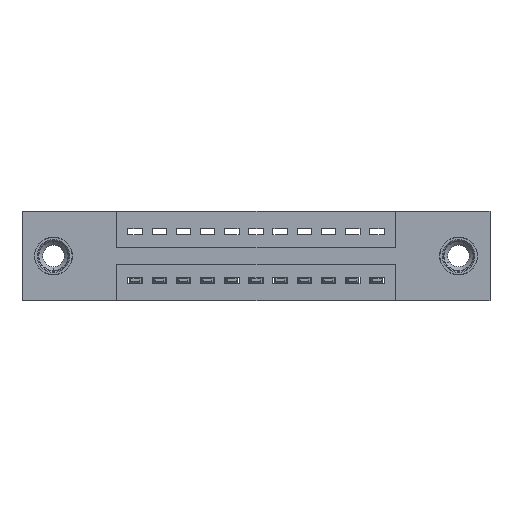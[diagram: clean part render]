
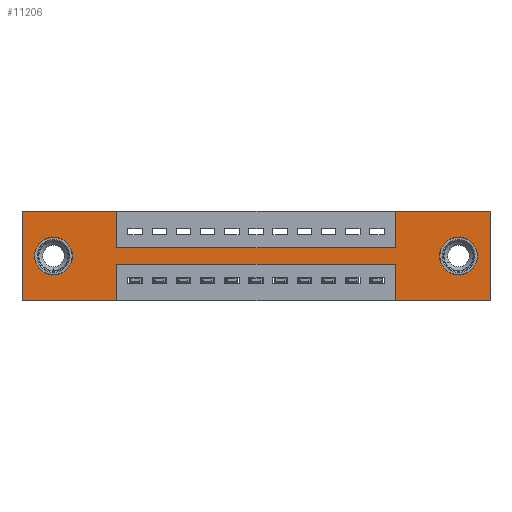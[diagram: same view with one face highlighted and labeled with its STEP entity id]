
A CAD part, front view. The second image highlights one B-rep face of the part: STEP entity #11206.
In plain terms, the highlighted planar face has unit normal (0, -1, 0).
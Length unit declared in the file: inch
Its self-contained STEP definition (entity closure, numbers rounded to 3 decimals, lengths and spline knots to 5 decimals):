
#356 = DIRECTION ( 'NONE',  ( -1., 0., 0. ) ) ;
#360 = ORIENTED_EDGE ( 'NONE', *, *, #8458, .F. ) ;
#380 = LINE ( 'NONE', #4766, #1817 ) ;
#430 = DIRECTION ( 'NONE',  ( 0., 1., 0. ) ) ;
#636 = ORIENTED_EDGE ( 'NONE', *, *, #5639, .F. ) ;
#683 = DIRECTION ( 'NONE',  ( 0., 0., -1. ) ) ;
#984 = CARTESIAN_POINT ( 'NONE',  ( 0.13, 0., -0.263 ) ) ;
#1240 = VERTEX_POINT ( 'NONE', #5807 ) ;
#1461 = VERTEX_POINT ( 'NONE', #5908 ) ;
#1475 = ORIENTED_EDGE ( 'NONE', *, *, #4261, .F. ) ;
#1483 = LINE ( 'NONE', #5819, #6664 ) ;
#1589 = EDGE_CURVE ( 'NONE', #9004, #10966, #3359, .T. ) ;
#1738 = VECTOR ( 'NONE', #13070, 39.37008 ) ;
#1817 = VECTOR ( 'NONE', #9837, 39.37008 ) ;
#1819 = EDGE_CURVE ( 'NONE', #8498, #11191, #4679, .T. ) ;
#1848 = FACE_BOUND ( 'NONE', #7551, .T. ) ;
#1968 = LINE ( 'NONE', #8083, #6820 ) ;
#1998 = ORIENTED_EDGE ( 'NONE', *, *, #6549, .F. ) ;
#2251 = VERTEX_POINT ( 'NONE', #9491 ) ;
#2304 = CARTESIAN_POINT ( 'NONE',  ( 0.3925, 0., -0.22 ) ) ;
#2522 = FACE_BOUND ( 'NONE', #7835, .T. ) ;
#2549 = VERTEX_POINT ( 'NONE', #10984 ) ;
#2738 = CARTESIAN_POINT ( 'NONE',  ( 1.935, 0., 0. ) ) ;
#3197 = PLANE ( 'NONE',  #4906 ) ;
#3282 = DIRECTION ( 'NONE',  ( -1., 0., 0. ) ) ;
#3312 = LINE ( 'NONE', #2304, #10624 ) ;
#3359 = LINE ( 'NONE', #5860, #1738 ) ;
#3496 = CARTESIAN_POINT ( 'NONE',  ( 1.805, 0., -0.107 ) ) ;
#3548 = DIRECTION ( 'NONE',  ( 0., 0., 1. ) ) ;
#3571 = ORIENTED_EDGE ( 'NONE', *, *, #1589, .F. ) ;
#4129 = CIRCLE ( 'NONE', #7503, 0.078 ) ;
#4219 = CARTESIAN_POINT ( 'NONE',  ( 0., 0., -0.37 ) ) ;
#4261 = EDGE_CURVE ( 'NONE', #1461, #6462, #380, .T. ) ;
#4270 = DIRECTION ( 'NONE',  ( 0., -1., 0. ) ) ;
#4402 = CARTESIAN_POINT ( 'NONE',  ( 0.3925, 0., 0. ) ) ;
#4442 = VECTOR ( 'NONE', #5449, 39.37008 ) ;
#4548 = DIRECTION ( 'NONE',  ( 0., 0., -1. ) ) ;
#4679 = CIRCLE ( 'NONE', #10626, 0.078 ) ;
#4725 = VECTOR ( 'NONE', #4548, 39.37008 ) ;
#4766 = CARTESIAN_POINT ( 'NONE',  ( 0., 0., 0. ) ) ;
#4904 = ORIENTED_EDGE ( 'NONE', *, *, #4978, .T. ) ;
#4906 = AXIS2_PLACEMENT_3D ( 'NONE', #10475, #4270, #11532 ) ;
#4953 = VECTOR ( 'NONE', #356, 39.37008 ) ;
#4954 = VECTOR ( 'NONE', #12612, 39.37008 ) ;
#4967 = CIRCLE ( 'NONE', #12934, 0.078 ) ;
#4978 = EDGE_CURVE ( 'NONE', #10634, #2251, #4129, .T. ) ;
#5097 = VERTEX_POINT ( 'NONE', #6298 ) ;
#5151 = CARTESIAN_POINT ( 'NONE',  ( 1.805, 0., -0.263 ) ) ;
#5184 = VERTEX_POINT ( 'NONE', #11077 ) ;
#5257 = DIRECTION ( 'NONE',  ( 0., 0., 1. ) ) ;
#5449 = DIRECTION ( 'NONE',  ( 0., 0., -1. ) ) ;
#5511 = ORIENTED_EDGE ( 'NONE', *, *, #7970, .F. ) ;
#5639 = EDGE_CURVE ( 'NONE', #10966, #6161, #13243, .T. ) ;
#5807 = CARTESIAN_POINT ( 'NONE',  ( 1.5425, 0., -0.37 ) ) ;
#5819 = CARTESIAN_POINT ( 'NONE',  ( 0., 0., 0. ) ) ;
#5829 = ORIENTED_EDGE ( 'NONE', *, *, #12043, .T. ) ;
#5836 = LINE ( 'NONE', #10740, #4725 ) ;
#5860 = CARTESIAN_POINT ( 'NONE',  ( 0.3925, 0., -0.37 ) ) ;
#5908 = CARTESIAN_POINT ( 'NONE',  ( 0., 0., 0. ) ) ;
#6161 = VERTEX_POINT ( 'NONE', #8451 ) ;
#6214 = LINE ( 'NONE', #4219, #4954 ) ;
#6296 = VERTEX_POINT ( 'NONE', #7533 ) ;
#6298 = CARTESIAN_POINT ( 'NONE',  ( 1.935, 0., -0.37 ) ) ;
#6394 = ORIENTED_EDGE ( 'NONE', *, *, #7751, .F. ) ;
#6450 = LINE ( 'NONE', #9413, #8413 ) ;
#6462 = VERTEX_POINT ( 'NONE', #11830 ) ;
#6549 = EDGE_CURVE ( 'NONE', #6161, #1461, #1968, .T. ) ;
#6664 = VECTOR ( 'NONE', #13110, 39.37008 ) ;
#6765 = VECTOR ( 'NONE', #5257, 39.37008 ) ;
#6820 = VECTOR ( 'NONE', #9135, 39.37008 ) ;
#6829 = ORIENTED_EDGE ( 'NONE', *, *, #9706, .F. ) ;
#7006 = EDGE_CURVE ( 'NONE', #2251, #10634, #13032, .T. ) ;
#7265 = CARTESIAN_POINT ( 'NONE',  ( 1.5425, 0., 0. ) ) ;
#7373 = ORIENTED_EDGE ( 'NONE', *, *, #13095, .F. ) ;
#7503 = AXIS2_PLACEMENT_3D ( 'NONE', #12890, #430, #3548 ) ;
#7533 = CARTESIAN_POINT ( 'NONE',  ( 1.5425, 0., 0. ) ) ;
#7551 = EDGE_LOOP ( 'NONE', ( #10809, #4904 ) ) ;
#7616 = DIRECTION ( 'NONE',  ( 0., 1., 0. ) ) ;
#7644 = EDGE_LOOP ( 'NONE', ( #3571, #11677, #6829, #8722, #6394, #7373, #360, #5511, #10384, #1475, #1998, #636 ) ) ;
#7751 = EDGE_CURVE ( 'NONE', #11159, #5097, #5836, .T. ) ;
#7835 = EDGE_LOOP ( 'NONE', ( #13031, #5829 ) ) ;
#7970 = EDGE_CURVE ( 'NONE', #5184, #12157, #6450, .T. ) ;
#8083 = CARTESIAN_POINT ( 'NONE',  ( 0., 0., 0. ) ) ;
#8365 = VECTOR ( 'NONE', #11875, 39.37008 ) ;
#8413 = VECTOR ( 'NONE', #10231, 39.37008 ) ;
#8451 = CARTESIAN_POINT ( 'NONE',  ( 0., 0., -0.37 ) ) ;
#8458 = EDGE_CURVE ( 'NONE', #12157, #6296, #11837, .T. ) ;
#8498 = VERTEX_POINT ( 'NONE', #3496 ) ;
#8528 = DIRECTION ( 'NONE',  ( 0., 0., -1. ) ) ;
#8722 = ORIENTED_EDGE ( 'NONE', *, *, #12394, .F. ) ;
#8934 = CARTESIAN_POINT ( 'NONE',  ( 1.5425, 0., -0.15 ) ) ;
#9004 = VERTEX_POINT ( 'NONE', #13440 ) ;
#9135 = DIRECTION ( 'NONE',  ( 0., 0., 1. ) ) ;
#9413 = CARTESIAN_POINT ( 'NONE',  ( 0.3925, 0., -0.15 ) ) ;
#9451 = CARTESIAN_POINT ( 'NONE',  ( 0.13, 0., -0.185 ) ) ;
#9491 = CARTESIAN_POINT ( 'NONE',  ( 0.13, 0., -0.107 ) ) ;
#9600 = CARTESIAN_POINT ( 'NONE',  ( 0.3925, 0., -0.37 ) ) ;
#9706 = EDGE_CURVE ( 'NONE', #1240, #2549, #12804, .T. ) ;
#9837 = DIRECTION ( 'NONE',  ( 1., 0., 0. ) ) ;
#9955 = CARTESIAN_POINT ( 'NONE',  ( 1.5425, 0., -0.37 ) ) ;
#10231 = DIRECTION ( 'NONE',  ( 1., 0., 0. ) ) ;
#10384 = ORIENTED_EDGE ( 'NONE', *, *, #12598, .F. ) ;
#10475 = CARTESIAN_POINT ( 'NONE',  ( 0., 0., -0.37 ) ) ;
#10624 = VECTOR ( 'NONE', #3282, 39.37008 ) ;
#10626 = AXIS2_PLACEMENT_3D ( 'NONE', #11067, #10929, #683 ) ;
#10634 = VERTEX_POINT ( 'NONE', #984 ) ;
#10740 = CARTESIAN_POINT ( 'NONE',  ( 1.935, 0., 0. ) ) ;
#10809 = ORIENTED_EDGE ( 'NONE', *, *, #7006, .T. ) ;
#10870 = EDGE_CURVE ( 'NONE', #2549, #9004, #3312, .T. ) ;
#10929 = DIRECTION ( 'NONE',  ( 0., 1., 0. ) ) ;
#10966 = VERTEX_POINT ( 'NONE', #9600 ) ;
#10984 = CARTESIAN_POINT ( 'NONE',  ( 1.5425, 0., -0.22 ) ) ;
#11067 = CARTESIAN_POINT ( 'NONE',  ( 1.805, 0., -0.185 ) ) ;
#11077 = CARTESIAN_POINT ( 'NONE',  ( 0.3925, 0., -0.15 ) ) ;
#11159 = VERTEX_POINT ( 'NONE', #2738 ) ;
#11191 = VERTEX_POINT ( 'NONE', #5151 ) ;
#11206 = ADVANCED_FACE ( 'NONE', ( #2522, #1848, #13263 ), #3197, .T. ) ;
#11532 = DIRECTION ( 'NONE',  ( 0., 0., -1. ) ) ;
#11607 = CARTESIAN_POINT ( 'NONE',  ( 0., 0., -0.37 ) ) ;
#11626 = DIRECTION ( 'NONE',  ( 0., 1., 0. ) ) ;
#11666 = CARTESIAN_POINT ( 'NONE',  ( 1.805, 0., -0.185 ) ) ;
#11677 = ORIENTED_EDGE ( 'NONE', *, *, #10870, .F. ) ;
#11830 = CARTESIAN_POINT ( 'NONE',  ( 0.3925, 0., 0. ) ) ;
#11837 = LINE ( 'NONE', #7265, #6765 ) ;
#11875 = DIRECTION ( 'NONE',  ( 0., 0., 1. ) ) ;
#11914 = LINE ( 'NONE', #4402, #4442 ) ;
#12007 = AXIS2_PLACEMENT_3D ( 'NONE', #9451, #11626, #12716 ) ;
#12043 = EDGE_CURVE ( 'NONE', #11191, #8498, #4967, .T. ) ;
#12157 = VERTEX_POINT ( 'NONE', #8934 ) ;
#12394 = EDGE_CURVE ( 'NONE', #5097, #1240, #6214, .T. ) ;
#12598 = EDGE_CURVE ( 'NONE', #6462, #5184, #11914, .T. ) ;
#12612 = DIRECTION ( 'NONE',  ( -1., 0., 0. ) ) ;
#12716 = DIRECTION ( 'NONE',  ( 0., 0., 1. ) ) ;
#12804 = LINE ( 'NONE', #9955, #8365 ) ;
#12890 = CARTESIAN_POINT ( 'NONE',  ( 0.13, 0., -0.185 ) ) ;
#12934 = AXIS2_PLACEMENT_3D ( 'NONE', #11666, #7616, #8528 ) ;
#13031 = ORIENTED_EDGE ( 'NONE', *, *, #1819, .T. ) ;
#13032 = CIRCLE ( 'NONE', #12007, 0.078 ) ;
#13070 = DIRECTION ( 'NONE',  ( 0., 0., -1. ) ) ;
#13095 = EDGE_CURVE ( 'NONE', #6296, #11159, #1483, .T. ) ;
#13110 = DIRECTION ( 'NONE',  ( 1., 0., 0. ) ) ;
#13243 = LINE ( 'NONE', #11607, #4953 ) ;
#13263 = FACE_OUTER_BOUND ( 'NONE', #7644, .T. ) ;
#13440 = CARTESIAN_POINT ( 'NONE',  ( 0.3925, 0., -0.22 ) ) ;
